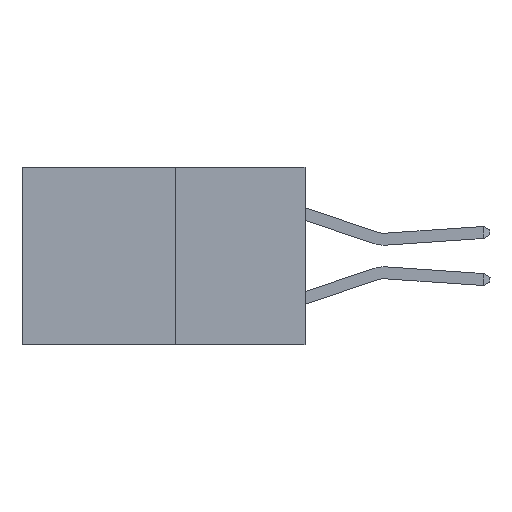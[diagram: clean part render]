
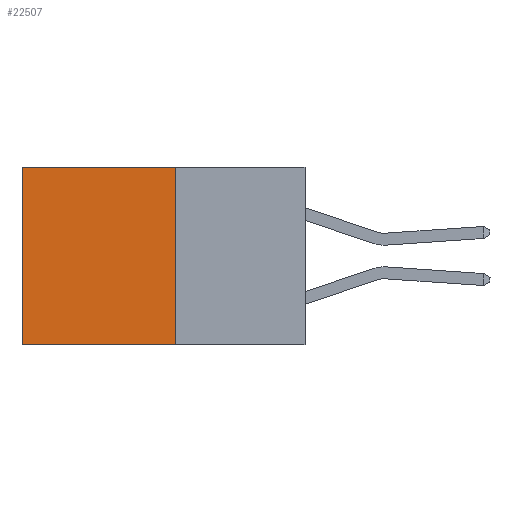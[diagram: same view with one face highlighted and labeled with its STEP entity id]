
A CAD part, left-side view. The second image highlights one B-rep face of the part: STEP entity #22507.
In plain terms, the highlighted planar face has unit normal (-1, 0, 0).
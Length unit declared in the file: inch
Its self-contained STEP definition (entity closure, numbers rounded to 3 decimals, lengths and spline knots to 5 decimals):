
#2392 = CARTESIAN_POINT ( 'NONE',  ( 0.277, 0.27, -0.37 ) ) ;
#2644 = AXIS2_PLACEMENT_3D ( 'NONE', #13780, #3349, #21695 ) ;
#2995 = CARTESIAN_POINT ( 'NONE',  ( 0.277, 0.27, 0. ) ) ;
#3349 = DIRECTION ( 'NONE',  ( 1., 0., 0. ) ) ;
#4255 = CARTESIAN_POINT ( 'NONE',  ( 0.277, 0.27, 0. ) ) ;
#5186 = EDGE_LOOP ( 'NONE', ( #14607, #26974, #23790, #30366 ) ) ;
#5291 = DIRECTION ( 'NONE',  ( 0., 0., -1. ) ) ;
#6901 = VERTEX_POINT ( 'NONE', #2995 ) ;
#10652 = CARTESIAN_POINT ( 'NONE',  ( 0.277, 0.59, -0.37 ) ) ;
#11314 = LINE ( 'NONE', #13209, #31309 ) ;
#11591 = LINE ( 'NONE', #30806, #17726 ) ;
#12231 = CARTESIAN_POINT ( 'NONE',  ( 0.277, 0.59, 0. ) ) ;
#12720 = EDGE_CURVE ( 'NONE', #6901, #22981, #11591, .T. ) ;
#13209 = CARTESIAN_POINT ( 'NONE',  ( 0.277, 0.59, -0.37 ) ) ;
#13345 = FACE_OUTER_BOUND ( 'NONE', #5186, .T. ) ;
#13780 = CARTESIAN_POINT ( 'NONE',  ( 0.277, 0.27, -0.37 ) ) ;
#14607 = ORIENTED_EDGE ( 'NONE', *, *, #22342, .T. ) ;
#16418 = PLANE ( 'NONE',  #2644 ) ;
#17726 = VECTOR ( 'NONE', #17812, 39.37008 ) ;
#17812 = DIRECTION ( 'NONE',  ( 0., 0., -1. ) ) ;
#20156 = LINE ( 'NONE', #4255, #33144 ) ;
#20750 = CARTESIAN_POINT ( 'NONE',  ( 0.277, 0.27, -0.37 ) ) ;
#21476 = VERTEX_POINT ( 'NONE', #10652 ) ;
#21695 = DIRECTION ( 'NONE',  ( 0., 0., -1. ) ) ;
#21896 = VERTEX_POINT ( 'NONE', #12231 ) ;
#22342 = EDGE_CURVE ( 'NONE', #21896, #21476, #11314, .T. ) ;
#22507 = ADVANCED_FACE ( 'NONE', ( #13345 ), #16418, .F. ) ;
#22795 = VECTOR ( 'NONE', #23464, 39.37008 ) ;
#22981 = VERTEX_POINT ( 'NONE', #2392 ) ;
#23464 = DIRECTION ( 'NONE',  ( 0., 1., 0. ) ) ;
#23790 = ORIENTED_EDGE ( 'NONE', *, *, #12720, .F. ) ;
#24758 = EDGE_CURVE ( 'NONE', #6901, #21896, #20156, .T. ) ;
#26974 = ORIENTED_EDGE ( 'NONE', *, *, #32243, .F. ) ;
#29740 = LINE ( 'NONE', #20750, #22795 ) ;
#30366 = ORIENTED_EDGE ( 'NONE', *, *, #24758, .T. ) ;
#30806 = CARTESIAN_POINT ( 'NONE',  ( 0.277, 0.27, -0.37 ) ) ;
#31309 = VECTOR ( 'NONE', #5291, 39.37008 ) ;
#32243 = EDGE_CURVE ( 'NONE', #22981, #21476, #29740, .T. ) ;
#33023 = DIRECTION ( 'NONE',  ( 0., 1., 0. ) ) ;
#33144 = VECTOR ( 'NONE', #33023, 39.37008 ) ;
